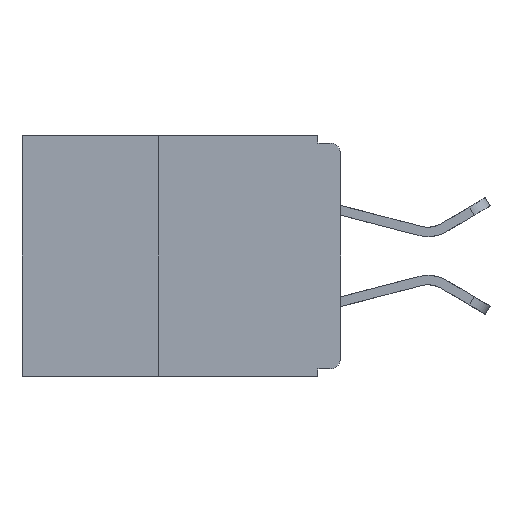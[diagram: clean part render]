
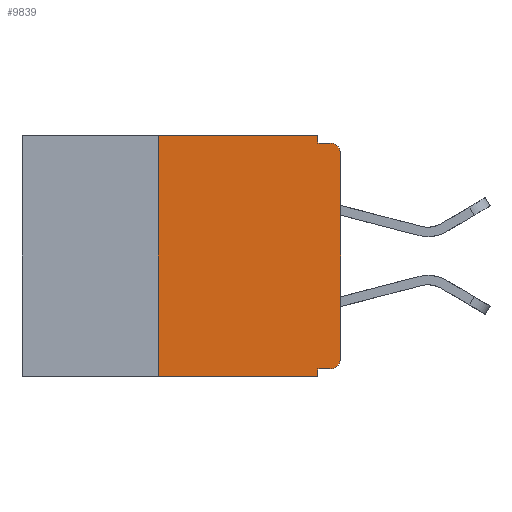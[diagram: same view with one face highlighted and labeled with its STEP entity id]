
A CAD part, left-side view. The second image highlights one B-rep face of the part: STEP entity #9839.
In plain terms, the highlighted planar face has unit normal (-1, 0, 0).
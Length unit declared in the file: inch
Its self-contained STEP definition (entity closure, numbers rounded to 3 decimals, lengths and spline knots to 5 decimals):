
#187 = VECTOR ( 'NONE', #1804, 39.37008 ) ;
#224 = CARTESIAN_POINT ( 'NONE',  ( 0., 0.031, -0.33 ) ) ;
#236 = VECTOR ( 'NONE', #15567, 39.37008 ) ;
#492 = CARTESIAN_POINT ( 'NONE',  ( 0., 0.437, 0. ) ) ;
#621 = VERTEX_POINT ( 'NONE', #4350 ) ;
#627 = CARTESIAN_POINT ( 'NONE',  ( 0., 0., 0. ) ) ;
#683 = CARTESIAN_POINT ( 'NONE',  ( 0., 0.015, -0.305 ) ) ;
#858 = DIRECTION ( 'NONE',  ( 0., 1., 0. ) ) ;
#1063 = VECTOR ( 'NONE', #12955, 39.37008 ) ;
#1483 = VERTEX_POINT ( 'NONE', #11071 ) ;
#1804 = DIRECTION ( 'NONE',  ( 0., -1., 0. ) ) ;
#1857 = LINE ( 'NONE', #4011, #4724 ) ;
#1940 = DIRECTION ( 'NONE',  ( 0., 0., -1. ) ) ;
#2071 = CARTESIAN_POINT ( 'NONE',  ( 0., 0.437, 0. ) ) ;
#2158 = CARTESIAN_POINT ( 'NONE',  ( 0., 0., -0.01 ) ) ;
#2300 = VERTEX_POINT ( 'NONE', #7415 ) ;
#2793 = EDGE_CURVE ( 'NONE', #11378, #2300, #10027, .T. ) ;
#3664 = CARTESIAN_POINT ( 'NONE',  ( 0., 0.015, -0.025 ) ) ;
#3984 = VERTEX_POINT ( 'NONE', #11460 ) ;
#4011 = CARTESIAN_POINT ( 'NONE',  ( 0., 0.437, -0.33 ) ) ;
#4219 = DIRECTION ( 'NONE',  ( 1., 0., 0. ) ) ;
#4350 = CARTESIAN_POINT ( 'NONE',  ( 0., 0., -0.025 ) ) ;
#4354 = CIRCLE ( 'NONE', #11679, 0.015 ) ;
#4724 = VECTOR ( 'NONE', #12638, 39.37008 ) ;
#4755 = LINE ( 'NONE', #8424, #8045 ) ;
#4776 = VERTEX_POINT ( 'NONE', #7162 ) ;
#4847 = EDGE_CURVE ( 'NONE', #621, #1483, #10324, .T. ) ;
#4906 = DIRECTION ( 'NONE',  ( 0., 0., -1. ) ) ;
#5730 = CARTESIAN_POINT ( 'NONE',  ( 0., 0.015, -0.32 ) ) ;
#5743 = ORIENTED_EDGE ( 'NONE', *, *, #14824, .T. ) ;
#5793 = AXIS2_PLACEMENT_3D ( 'NONE', #3664, #12263, #4906 ) ;
#5851 = DIRECTION ( 'NONE',  ( 0., -1., 0. ) ) ;
#6066 = LINE ( 'NONE', #2158, #9367 ) ;
#7162 = CARTESIAN_POINT ( 'NONE',  ( 0., 0.031, -0.32 ) ) ;
#7415 = CARTESIAN_POINT ( 'NONE',  ( 0., 0.031, 0. ) ) ;
#7865 = CARTESIAN_POINT ( 'NONE',  ( 0., 0.031, 0. ) ) ;
#8045 = VECTOR ( 'NONE', #858, 39.37008 ) ;
#8276 = ORIENTED_EDGE ( 'NONE', *, *, #12908, .F. ) ;
#8424 = CARTESIAN_POINT ( 'NONE',  ( 0., 0., -0.32 ) ) ;
#9318 = DIRECTION ( 'NONE',  ( -1., 0., 0. ) ) ;
#9331 = FACE_OUTER_BOUND ( 'NONE', #9885, .T. ) ;
#9367 = VECTOR ( 'NONE', #5851, 39.37008 ) ;
#9469 = VECTOR ( 'NONE', #11560, 39.37008 ) ;
#9608 = ORIENTED_EDGE ( 'NONE', *, *, #14934, .F. ) ;
#9839 = ADVANCED_FACE ( 'NONE', ( #9331 ), #11582, .F. ) ;
#9885 = EDGE_LOOP ( 'NONE', ( #5743, #13827, #9608, #13255, #14395, #8276, #15879, #13080, #14586, #12104 ) ) ;
#9942 = VERTEX_POINT ( 'NONE', #13750 ) ;
#10027 = LINE ( 'NONE', #2071, #187 ) ;
#10186 = LINE ( 'NONE', #10595, #12706 ) ;
#10240 = EDGE_CURVE ( 'NONE', #4776, #15775, #13325, .T. ) ;
#10324 = CIRCLE ( 'NONE', #5793, 0.015 ) ;
#10595 = CARTESIAN_POINT ( 'NONE',  ( 0., 0.25, -0.33 ) ) ;
#11071 = CARTESIAN_POINT ( 'NONE',  ( 0., 0.015, -0.01 ) ) ;
#11353 = EDGE_CURVE ( 'NONE', #2300, #12501, #12731, .T. ) ;
#11378 = VERTEX_POINT ( 'NONE', #15233 ) ;
#11460 = CARTESIAN_POINT ( 'NONE',  ( 0., 0., -0.305 ) ) ;
#11523 = AXIS2_PLACEMENT_3D ( 'NONE', #492, #4219, #12828 ) ;
#11560 = DIRECTION ( 'NONE',  ( 0., 0., -1. ) ) ;
#11582 = PLANE ( 'NONE',  #11523 ) ;
#11679 = AXIS2_PLACEMENT_3D ( 'NONE', #683, #9318, #1940 ) ;
#11773 = DIRECTION ( 'NONE',  ( 0., 0., 1. ) ) ;
#11903 = CARTESIAN_POINT ( 'NONE',  ( 0., 0.031, -0.33 ) ) ;
#12104 = ORIENTED_EDGE ( 'NONE', *, *, #14834, .T. ) ;
#12201 = VERTEX_POINT ( 'NONE', #5730 ) ;
#12263 = DIRECTION ( 'NONE',  ( -1., 0., 0. ) ) ;
#12501 = VERTEX_POINT ( 'NONE', #12508 ) ;
#12508 = CARTESIAN_POINT ( 'NONE',  ( 0., 0.031, -0.01 ) ) ;
#12638 = DIRECTION ( 'NONE',  ( 0., -1., 0. ) ) ;
#12706 = VECTOR ( 'NONE', #11773, 39.37008 ) ;
#12731 = LINE ( 'NONE', #7865, #9469 ) ;
#12828 = DIRECTION ( 'NONE',  ( 0., 0., -1. ) ) ;
#12908 = EDGE_CURVE ( 'NONE', #9942, #11378, #10186, .T. ) ;
#12955 = DIRECTION ( 'NONE',  ( 0., 0., 1. ) ) ;
#13080 = ORIENTED_EDGE ( 'NONE', *, *, #10240, .F. ) ;
#13255 = ORIENTED_EDGE ( 'NONE', *, *, #11353, .F. ) ;
#13325 = LINE ( 'NONE', #11903, #236 ) ;
#13750 = CARTESIAN_POINT ( 'NONE',  ( 0., 0.25, -0.33 ) ) ;
#13827 = ORIENTED_EDGE ( 'NONE', *, *, #4847, .T. ) ;
#14395 = ORIENTED_EDGE ( 'NONE', *, *, #2793, .F. ) ;
#14396 = EDGE_CURVE ( 'NONE', #12201, #4776, #4755, .T. ) ;
#14526 = LINE ( 'NONE', #627, #1063 ) ;
#14586 = ORIENTED_EDGE ( 'NONE', *, *, #14396, .F. ) ;
#14824 = EDGE_CURVE ( 'NONE', #3984, #621, #14526, .T. ) ;
#14834 = EDGE_CURVE ( 'NONE', #12201, #3984, #4354, .T. ) ;
#14934 = EDGE_CURVE ( 'NONE', #12501, #1483, #6066, .T. ) ;
#15233 = CARTESIAN_POINT ( 'NONE',  ( 0., 0.25, 0. ) ) ;
#15243 = EDGE_CURVE ( 'NONE', #9942, #15775, #1857, .T. ) ;
#15567 = DIRECTION ( 'NONE',  ( 0., 0., -1. ) ) ;
#15775 = VERTEX_POINT ( 'NONE', #224 ) ;
#15879 = ORIENTED_EDGE ( 'NONE', *, *, #15243, .T. ) ;
